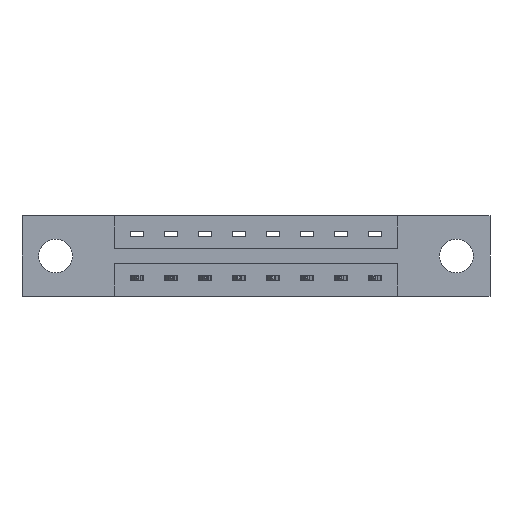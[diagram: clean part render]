
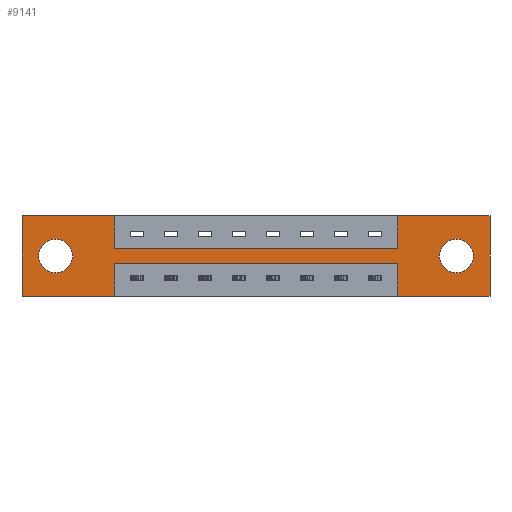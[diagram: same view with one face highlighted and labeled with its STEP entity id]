
A CAD part, front view. The second image highlights one B-rep face of the part: STEP entity #9141.
In plain terms, the highlighted planar face has unit normal (0, -1, 0).
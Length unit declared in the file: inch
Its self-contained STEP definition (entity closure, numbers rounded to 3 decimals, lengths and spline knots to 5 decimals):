
#209 = VECTOR ( 'NONE', #1234, 39.37008 ) ;
#217 = DIRECTION ( 'NONE',  ( 0., 0., -1. ) ) ;
#230 = VECTOR ( 'NONE', #7975, 39.37008 ) ;
#235 = CARTESIAN_POINT ( 'NONE',  ( 0.425, 0., 0. ) ) ;
#344 = EDGE_LOOP ( 'NONE', ( #7807, #7093 ) ) ;
#593 = EDGE_CURVE ( 'NONE', #3036, #6008, #7545, .T. ) ;
#609 = CARTESIAN_POINT ( 'NONE',  ( 0.155, 0., -0.107 ) ) ;
#788 = CARTESIAN_POINT ( 'NONE',  ( 0.155, 0., -0.263 ) ) ;
#800 = CARTESIAN_POINT ( 'NONE',  ( 0.155, 0., -0.185 ) ) ;
#816 = ORIENTED_EDGE ( 'NONE', *, *, #9633, .F. ) ;
#923 = VERTEX_POINT ( 'NONE', #609 ) ;
#1087 = FACE_BOUND ( 'NONE', #10253, .T. ) ;
#1230 = CARTESIAN_POINT ( 'NONE',  ( 0., 0., 0. ) ) ;
#1234 = DIRECTION ( 'NONE',  ( -1., 0., 0. ) ) ;
#1237 = DIRECTION ( 'NONE',  ( 0., 0., 1. ) ) ;
#1254 = VECTOR ( 'NONE', #1237, 39.37008 ) ;
#1296 = CARTESIAN_POINT ( 'NONE',  ( 1.729, 0., 0. ) ) ;
#1348 = DIRECTION ( 'NONE',  ( 0., 0., -1. ) ) ;
#1378 = AXIS2_PLACEMENT_3D ( 'NONE', #10178, #5309, #1348 ) ;
#1500 = DIRECTION ( 'NONE',  ( 0., 1., 0. ) ) ;
#1508 = VERTEX_POINT ( 'NONE', #1965 ) ;
#1823 = LINE ( 'NONE', #9723, #5796 ) ;
#1965 = CARTESIAN_POINT ( 'NONE',  ( 1.729, 0., -0.22 ) ) ;
#1996 = DIRECTION ( 'NONE',  ( 0., 0., 1. ) ) ;
#2110 = DIRECTION ( 'NONE',  ( 1., 0., 0. ) ) ;
#2372 = CARTESIAN_POINT ( 'NONE',  ( 0.425, 0., -0.22 ) ) ;
#2430 = VECTOR ( 'NONE', #9783, 39.37008 ) ;
#2466 = DIRECTION ( 'NONE',  ( 0., 0., -1. ) ) ;
#2471 = ORIENTED_EDGE ( 'NONE', *, *, #593, .F. ) ;
#2652 = VERTEX_POINT ( 'NONE', #9033 ) ;
#2739 = EDGE_CURVE ( 'NONE', #6091, #9840, #10109, .T. ) ;
#2809 = LINE ( 'NONE', #3722, #6532 ) ;
#2945 = VERTEX_POINT ( 'NONE', #4910 ) ;
#3036 = VERTEX_POINT ( 'NONE', #3770 ) ;
#3100 = DIRECTION ( 'NONE',  ( 0., 0., 1. ) ) ;
#3197 = EDGE_CURVE ( 'NONE', #7120, #6091, #6951, .T. ) ;
#3256 = EDGE_CURVE ( 'NONE', #1508, #8662, #8858, .T. ) ;
#3355 = VERTEX_POINT ( 'NONE', #4270 ) ;
#3399 = EDGE_CURVE ( 'NONE', #923, #8919, #7580, .T. ) ;
#3585 = EDGE_CURVE ( 'NONE', #9840, #2945, #9472, .T. ) ;
#3722 = CARTESIAN_POINT ( 'NONE',  ( 0., 0., -0.37 ) ) ;
#3770 = CARTESIAN_POINT ( 'NONE',  ( 0., 0., 0. ) ) ;
#3842 = VERTEX_POINT ( 'NONE', #8276 ) ;
#3946 = ORIENTED_EDGE ( 'NONE', *, *, #8688, .F. ) ;
#4111 = AXIS2_PLACEMENT_3D ( 'NONE', #10222, #8528, #4503 ) ;
#4228 = CARTESIAN_POINT ( 'NONE',  ( 0.155, 0., -0.185 ) ) ;
#4270 = CARTESIAN_POINT ( 'NONE',  ( 1.999, 0., -0.263 ) ) ;
#4317 = CARTESIAN_POINT ( 'NONE',  ( 0., 0., 0. ) ) ;
#4441 = CARTESIAN_POINT ( 'NONE',  ( 2.154, 0., 0. ) ) ;
#4451 = CARTESIAN_POINT ( 'NONE',  ( 0.425, 0., -0.22 ) ) ;
#4503 = DIRECTION ( 'NONE',  ( 0., 0., -1. ) ) ;
#4769 = CARTESIAN_POINT ( 'NONE',  ( 1.729, 0., 0. ) ) ;
#4821 = ORIENTED_EDGE ( 'NONE', *, *, #9869, .F. ) ;
#4833 = VECTOR ( 'NONE', #7547, 39.37008 ) ;
#4855 = CIRCLE ( 'NONE', #5041, 0.078 ) ;
#4910 = CARTESIAN_POINT ( 'NONE',  ( 1.729, 0., -0.37 ) ) ;
#4917 = EDGE_CURVE ( 'NONE', #3355, #3842, #9800, .T. ) ;
#5041 = AXIS2_PLACEMENT_3D ( 'NONE', #800, #1500, #3100 ) ;
#5058 = AXIS2_PLACEMENT_3D ( 'NONE', #9007, #8935, #217 ) ;
#5102 = CARTESIAN_POINT ( 'NONE',  ( 2.154, 0., -0.37 ) ) ;
#5103 = DIRECTION ( 'NONE',  ( 0., 0., 1. ) ) ;
#5108 = VERTEX_POINT ( 'NONE', #9729 ) ;
#5132 = EDGE_CURVE ( 'NONE', #6811, #9333, #6637, .T. ) ;
#5179 = LINE ( 'NONE', #6959, #7923 ) ;
#5188 = ORIENTED_EDGE ( 'NONE', *, *, #3197, .F. ) ;
#5259 = VECTOR ( 'NONE', #7146, 39.37008 ) ;
#5309 = DIRECTION ( 'NONE',  ( 0., 1., 0. ) ) ;
#5580 = DIRECTION ( 'NONE',  ( -1., 0., 0. ) ) ;
#5728 = ORIENTED_EDGE ( 'NONE', *, *, #3256, .F. ) ;
#5744 = PLANE ( 'NONE',  #5058 ) ;
#5759 = VECTOR ( 'NONE', #8033, 39.37008 ) ;
#5796 = VECTOR ( 'NONE', #2466, 39.37008 ) ;
#5838 = LINE ( 'NONE', #1296, #1254 ) ;
#5897 = AXIS2_PLACEMENT_3D ( 'NONE', #4228, #6714, #5103 ) ;
#5970 = EDGE_CURVE ( 'NONE', #5108, #3036, #6365, .T. ) ;
#6008 = VERTEX_POINT ( 'NONE', #235 ) ;
#6091 = VERTEX_POINT ( 'NONE', #4441 ) ;
#6092 = ORIENTED_EDGE ( 'NONE', *, *, #6194, .T. ) ;
#6119 = CARTESIAN_POINT ( 'NONE',  ( 0., 0., 0. ) ) ;
#6194 = EDGE_CURVE ( 'NONE', #3842, #3355, #9655, .T. ) ;
#6295 = CARTESIAN_POINT ( 'NONE',  ( 0., 0., -0.37 ) ) ;
#6365 = LINE ( 'NONE', #6119, #5259 ) ;
#6380 = ORIENTED_EDGE ( 'NONE', *, *, #10052, .F. ) ;
#6502 = CARTESIAN_POINT ( 'NONE',  ( 0.425, 0., -0.15 ) ) ;
#6532 = VECTOR ( 'NONE', #6780, 39.37008 ) ;
#6637 = LINE ( 'NONE', #6502, #5759 ) ;
#6714 = DIRECTION ( 'NONE',  ( 0., 1., 0. ) ) ;
#6780 = DIRECTION ( 'NONE',  ( -1., 0., 0. ) ) ;
#6811 = VERTEX_POINT ( 'NONE', #8021 ) ;
#6951 = LINE ( 'NONE', #4317, #4833 ) ;
#6959 = CARTESIAN_POINT ( 'NONE',  ( 1.729, 0., -0.37 ) ) ;
#7026 = EDGE_CURVE ( 'NONE', #9333, #7120, #5838, .T. ) ;
#7087 = EDGE_CURVE ( 'NONE', #8919, #923, #4855, .T. ) ;
#7093 = ORIENTED_EDGE ( 'NONE', *, *, #7087, .T. ) ;
#7120 = VERTEX_POINT ( 'NONE', #4769 ) ;
#7146 = DIRECTION ( 'NONE',  ( 0., 0., 1. ) ) ;
#7545 = LINE ( 'NONE', #1230, #9070 ) ;
#7547 = DIRECTION ( 'NONE',  ( 1., 0., 0. ) ) ;
#7578 = FACE_OUTER_BOUND ( 'NONE', #9827, .T. ) ;
#7580 = CIRCLE ( 'NONE', #5897, 0.078 ) ;
#7702 = FACE_BOUND ( 'NONE', #344, .T. ) ;
#7807 = ORIENTED_EDGE ( 'NONE', *, *, #3399, .T. ) ;
#7923 = VECTOR ( 'NONE', #1996, 39.37008 ) ;
#7975 = DIRECTION ( 'NONE',  ( 0., 0., -1. ) ) ;
#8021 = CARTESIAN_POINT ( 'NONE',  ( 0.425, 0., -0.15 ) ) ;
#8033 = DIRECTION ( 'NONE',  ( 1., 0., 0. ) ) ;
#8276 = CARTESIAN_POINT ( 'NONE',  ( 1.999, 0., -0.107 ) ) ;
#8528 = DIRECTION ( 'NONE',  ( 0., 1., 0. ) ) ;
#8662 = VERTEX_POINT ( 'NONE', #2372 ) ;
#8688 = EDGE_CURVE ( 'NONE', #8662, #2652, #1823, .T. ) ;
#8758 = CARTESIAN_POINT ( 'NONE',  ( 1.729, 0., -0.15 ) ) ;
#8799 = CARTESIAN_POINT ( 'NONE',  ( 2.154, 0., 0. ) ) ;
#8806 = ORIENTED_EDGE ( 'NONE', *, *, #4917, .T. ) ;
#8858 = LINE ( 'NONE', #4451, #209 ) ;
#8919 = VERTEX_POINT ( 'NONE', #788 ) ;
#8935 = DIRECTION ( 'NONE',  ( 0., -1., 0. ) ) ;
#9007 = CARTESIAN_POINT ( 'NONE',  ( 0., 0., -0.37 ) ) ;
#9033 = CARTESIAN_POINT ( 'NONE',  ( 0.425, 0., -0.37 ) ) ;
#9070 = VECTOR ( 'NONE', #2110, 39.37008 ) ;
#9141 = ADVANCED_FACE ( 'NONE', ( #1087, #7702, #7578 ), #5744, .T. ) ;
#9333 = VERTEX_POINT ( 'NONE', #8758 ) ;
#9464 = ORIENTED_EDGE ( 'NONE', *, *, #5132, .F. ) ;
#9472 = LINE ( 'NONE', #6295, #9956 ) ;
#9561 = ORIENTED_EDGE ( 'NONE', *, *, #2739, .F. ) ;
#9585 = LINE ( 'NONE', #9686, #2430 ) ;
#9633 = EDGE_CURVE ( 'NONE', #6008, #6811, #9585, .T. ) ;
#9655 = CIRCLE ( 'NONE', #1378, 0.078 ) ;
#9686 = CARTESIAN_POINT ( 'NONE',  ( 0.425, 0., 0. ) ) ;
#9723 = CARTESIAN_POINT ( 'NONE',  ( 0.425, 0., -0.37 ) ) ;
#9729 = CARTESIAN_POINT ( 'NONE',  ( 0., 0., -0.37 ) ) ;
#9783 = DIRECTION ( 'NONE',  ( 0., 0., -1. ) ) ;
#9800 = CIRCLE ( 'NONE', #4111, 0.078 ) ;
#9827 = EDGE_LOOP ( 'NONE', ( #3946, #5728, #6380, #9883, #9561, #5188, #9952, #9464, #816, #2471, #10151, #4821 ) ) ;
#9840 = VERTEX_POINT ( 'NONE', #5102 ) ;
#9869 = EDGE_CURVE ( 'NONE', #2652, #5108, #2809, .T. ) ;
#9883 = ORIENTED_EDGE ( 'NONE', *, *, #3585, .F. ) ;
#9952 = ORIENTED_EDGE ( 'NONE', *, *, #7026, .F. ) ;
#9956 = VECTOR ( 'NONE', #5580, 39.37008 ) ;
#10052 = EDGE_CURVE ( 'NONE', #2945, #1508, #5179, .T. ) ;
#10109 = LINE ( 'NONE', #8799, #230 ) ;
#10151 = ORIENTED_EDGE ( 'NONE', *, *, #5970, .F. ) ;
#10178 = CARTESIAN_POINT ( 'NONE',  ( 1.999, 0., -0.185 ) ) ;
#10222 = CARTESIAN_POINT ( 'NONE',  ( 1.999, 0., -0.185 ) ) ;
#10253 = EDGE_LOOP ( 'NONE', ( #6092, #8806 ) ) ;
